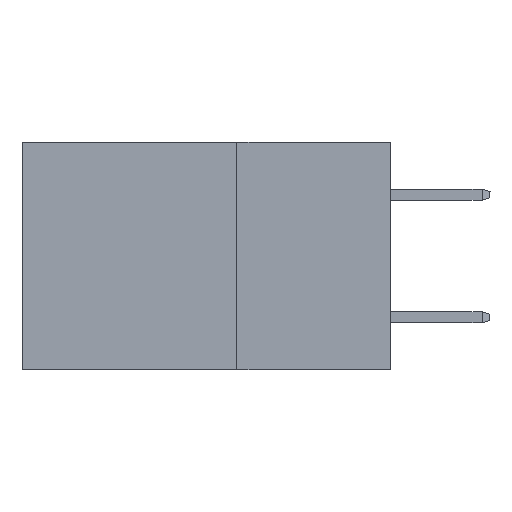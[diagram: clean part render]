
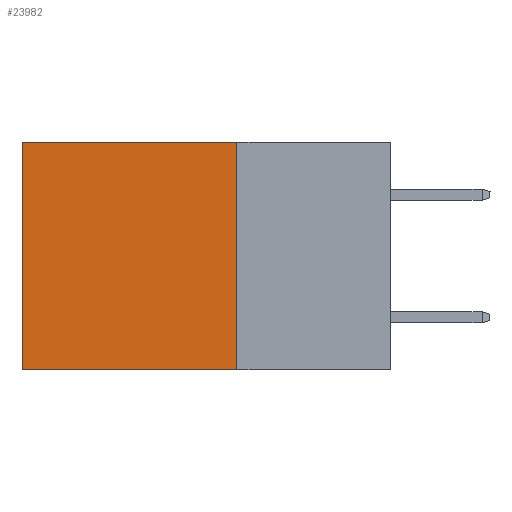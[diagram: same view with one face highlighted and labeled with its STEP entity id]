
A CAD part, left-side view. The second image highlights one B-rep face of the part: STEP entity #23982.
In plain terms, the highlighted planar face has unit normal (-1, 0, 0).
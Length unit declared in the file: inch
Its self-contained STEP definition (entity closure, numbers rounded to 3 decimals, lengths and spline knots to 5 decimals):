
#415 = LINE ( 'NONE', #12152, #11862 ) ;
#918 = CARTESIAN_POINT ( 'NONE',  ( 0.2875, 0.6, 0. ) ) ;
#1286 = DIRECTION ( 'NONE',  ( 0., 1., 0. ) ) ;
#2533 = CARTESIAN_POINT ( 'NONE',  ( 0.2875, 0.25, 0. ) ) ;
#3804 = DIRECTION ( 'NONE',  ( 0., 0., -1. ) ) ;
#4049 = PLANE ( 'NONE',  #9769 ) ;
#4174 = CARTESIAN_POINT ( 'NONE',  ( 0.2875, 0.25, 0. ) ) ;
#4216 = ORIENTED_EDGE ( 'NONE', *, *, #25362, .F. ) ;
#5837 = LINE ( 'NONE', #13516, #23303 ) ;
#6092 = VECTOR ( 'NONE', #14795, 39.37008 ) ;
#6247 = VERTEX_POINT ( 'NONE', #13501 ) ;
#6596 = EDGE_CURVE ( 'NONE', #9788, #6247, #10754, .T. ) ;
#7287 = EDGE_LOOP ( 'NONE', ( #25030, #13033, #4216, #18403 ) ) ;
#7862 = VERTEX_POINT ( 'NONE', #14526 ) ;
#9334 = EDGE_CURVE ( 'NONE', #6247, #20498, #18773, .T. ) ;
#9769 = AXIS2_PLACEMENT_3D ( 'NONE', #4174, #18128, #3804 ) ;
#9788 = VERTEX_POINT ( 'NONE', #23534 ) ;
#10754 = LINE ( 'NONE', #2533, #6092 ) ;
#11862 = VECTOR ( 'NONE', #15932, 39.37008 ) ;
#12152 = CARTESIAN_POINT ( 'NONE',  ( 0.2875, 0.25, 0. ) ) ;
#13033 = ORIENTED_EDGE ( 'NONE', *, *, #15093, .F. ) ;
#13501 = CARTESIAN_POINT ( 'NONE',  ( 0.2875, 0.6, 0. ) ) ;
#13516 = CARTESIAN_POINT ( 'NONE',  ( 0.2875, 0.25, -0.37 ) ) ;
#13657 = CARTESIAN_POINT ( 'NONE',  ( 0.2875, 0.6, -0.37 ) ) ;
#14526 = CARTESIAN_POINT ( 'NONE',  ( 0.2875, 0.25, -0.37 ) ) ;
#14795 = DIRECTION ( 'NONE',  ( 0., 1., 0. ) ) ;
#15093 = EDGE_CURVE ( 'NONE', #7862, #20498, #5837, .T. ) ;
#15932 = DIRECTION ( 'NONE',  ( 0., 0., -1. ) ) ;
#18128 = DIRECTION ( 'NONE',  ( 1., 0., 0. ) ) ;
#18403 = ORIENTED_EDGE ( 'NONE', *, *, #6596, .T. ) ;
#18773 = LINE ( 'NONE', #918, #19027 ) ;
#19027 = VECTOR ( 'NONE', #20590, 39.37008 ) ;
#19707 = FACE_OUTER_BOUND ( 'NONE', #7287, .T. ) ;
#20498 = VERTEX_POINT ( 'NONE', #13657 ) ;
#20590 = DIRECTION ( 'NONE',  ( 0., 0., -1. ) ) ;
#23303 = VECTOR ( 'NONE', #1286, 39.37008 ) ;
#23534 = CARTESIAN_POINT ( 'NONE',  ( 0.2875, 0.25, 0. ) ) ;
#23982 = ADVANCED_FACE ( 'NONE', ( #19707 ), #4049, .F. ) ;
#25030 = ORIENTED_EDGE ( 'NONE', *, *, #9334, .T. ) ;
#25362 = EDGE_CURVE ( 'NONE', #9788, #7862, #415, .T. ) ;
